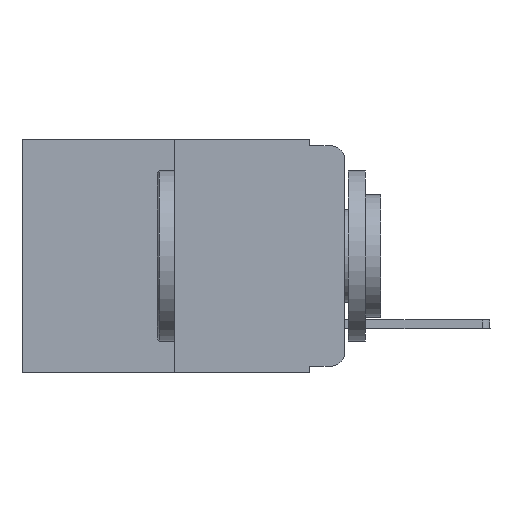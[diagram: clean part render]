
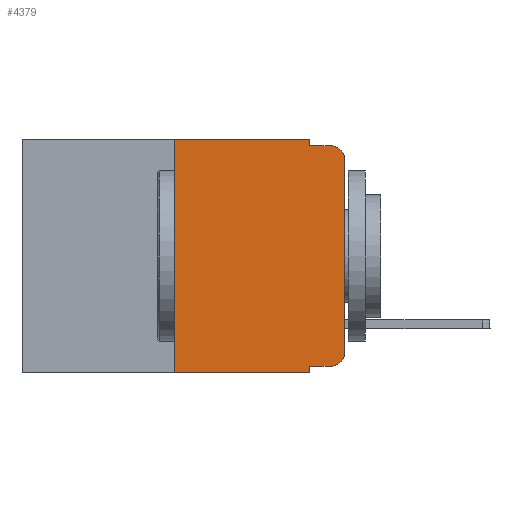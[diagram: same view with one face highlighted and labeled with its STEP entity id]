
A CAD part, left-side view. The second image highlights one B-rep face of the part: STEP entity #4379.
In plain terms, the highlighted planar face has unit normal (-1, 0, 0).
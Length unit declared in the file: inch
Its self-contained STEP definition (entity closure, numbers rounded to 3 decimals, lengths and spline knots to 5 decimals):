
#261 = DIRECTION ( 'NONE',  ( -1., 0., 0. ) ) ;
#300 = CARTESIAN_POINT ( 'NONE',  ( 0., 0.25, 0. ) ) ;
#353 = EDGE_CURVE ( 'NONE', #5328, #11144, #6289, .T. ) ;
#721 = VERTEX_POINT ( 'NONE', #13155 ) ;
#732 = LINE ( 'NONE', #4503, #10859 ) ;
#822 = ORIENTED_EDGE ( 'NONE', *, *, #2359, .T. ) ;
#826 = CARTESIAN_POINT ( 'NONE',  ( 0., 0.051, -0.01 ) ) ;
#854 = DIRECTION ( 'NONE',  ( 0., 0., -1. ) ) ;
#1128 = LINE ( 'NONE', #4908, #9444 ) ;
#1328 = DIRECTION ( 'NONE',  ( 0., 0., -1. ) ) ;
#1804 = VECTOR ( 'NONE', #5102, 39.37008 ) ;
#1822 = CARTESIAN_POINT ( 'NONE',  ( 0., 0.051, 0. ) ) ;
#1845 = FACE_OUTER_BOUND ( 'NONE', #6789, .T. ) ;
#1897 = DIRECTION ( 'NONE',  ( -1., 0., 0. ) ) ;
#2022 = VERTEX_POINT ( 'NONE', #10304 ) ;
#2359 = EDGE_CURVE ( 'NONE', #3665, #721, #9091, .T. ) ;
#2827 = ORIENTED_EDGE ( 'NONE', *, *, #7366, .F. ) ;
#2934 = DIRECTION ( 'NONE',  ( 0., 0., -1. ) ) ;
#3153 = VECTOR ( 'NONE', #10690, 39.37008 ) ;
#3536 = VECTOR ( 'NONE', #5840, 39.37008 ) ;
#3557 = CIRCLE ( 'NONE', #5397, 0.02 ) ;
#3665 = VERTEX_POINT ( 'NONE', #5564 ) ;
#3994 = DIRECTION ( 'NONE',  ( 1., 0., 0. ) ) ;
#4379 = ADVANCED_FACE ( 'NONE', ( #1845 ), #5975, .F. ) ;
#4503 = CARTESIAN_POINT ( 'NONE',  ( 0., 0.25, 0. ) ) ;
#4523 = DIRECTION ( 'NONE',  ( 0., -1., 0. ) ) ;
#4739 = CARTESIAN_POINT ( 'NONE',  ( 0., 0.051, 0. ) ) ;
#4783 = EDGE_CURVE ( 'NONE', #3665, #11144, #7653, .T. ) ;
#4908 = CARTESIAN_POINT ( 'NONE',  ( 0., 0., 0. ) ) ;
#5009 = CARTESIAN_POINT ( 'NONE',  ( 0., 0.051, -0.333 ) ) ;
#5102 = DIRECTION ( 'NONE',  ( 0., -1., 0. ) ) ;
#5114 = EDGE_CURVE ( 'NONE', #721, #13021, #11099, .T. ) ;
#5180 = CARTESIAN_POINT ( 'NONE',  ( 0., 0.473, 0. ) ) ;
#5328 = VERTEX_POINT ( 'NONE', #10017 ) ;
#5397 = AXIS2_PLACEMENT_3D ( 'NONE', #10200, #1897, #2934 ) ;
#5564 = CARTESIAN_POINT ( 'NONE',  ( 0., 0.051, -0.333 ) ) ;
#5840 = DIRECTION ( 'NONE',  ( 0., -1., 0. ) ) ;
#5975 = PLANE ( 'NONE',  #6290 ) ;
#6289 = LINE ( 'NONE', #8960, #3536 ) ;
#6290 = AXIS2_PLACEMENT_3D ( 'NONE', #5180, #3994, #854 ) ;
#6679 = EDGE_CURVE ( 'NONE', #7228, #2022, #3557, .T. ) ;
#6789 = EDGE_LOOP ( 'NONE', ( #12025, #11749, #9859, #8023, #7413, #2827, #7099, #11993, #822, #6969 ) ) ;
#6950 = CARTESIAN_POINT ( 'NONE',  ( 0., 0.051, -0.343 ) ) ;
#6969 = ORIENTED_EDGE ( 'NONE', *, *, #5114, .T. ) ;
#7013 = DIRECTION ( 'NONE',  ( 0., 0., 1. ) ) ;
#7099 = ORIENTED_EDGE ( 'NONE', *, *, #353, .T. ) ;
#7206 = VERTEX_POINT ( 'NONE', #1822 ) ;
#7228 = VERTEX_POINT ( 'NONE', #13267 ) ;
#7366 = EDGE_CURVE ( 'NONE', #5328, #9030, #732, .T. ) ;
#7413 = ORIENTED_EDGE ( 'NONE', *, *, #11383, .F. ) ;
#7653 = LINE ( 'NONE', #4739, #3153 ) ;
#7656 = EDGE_CURVE ( 'NONE', #9646, #2022, #9375, .T. ) ;
#8023 = ORIENTED_EDGE ( 'NONE', *, *, #13502, .F. ) ;
#8039 = CARTESIAN_POINT ( 'NONE',  ( 0., 0.02, -0.313 ) ) ;
#8700 = DIRECTION ( 'NONE',  ( 0., 0., 1. ) ) ;
#8789 = VECTOR ( 'NONE', #13421, 39.37008 ) ;
#8960 = CARTESIAN_POINT ( 'NONE',  ( 0., 0.473, -0.343 ) ) ;
#9030 = VERTEX_POINT ( 'NONE', #300 ) ;
#9080 = CARTESIAN_POINT ( 'NONE',  ( 0., 0.051, 0. ) ) ;
#9091 = LINE ( 'NONE', #5009, #1804 ) ;
#9375 = LINE ( 'NONE', #826, #10024 ) ;
#9444 = VECTOR ( 'NONE', #7013, 39.37008 ) ;
#9646 = VERTEX_POINT ( 'NONE', #11475 ) ;
#9859 = ORIENTED_EDGE ( 'NONE', *, *, #7656, .F. ) ;
#10017 = CARTESIAN_POINT ( 'NONE',  ( 0., 0.25, -0.343 ) ) ;
#10024 = VECTOR ( 'NONE', #13308, 39.37008 ) ;
#10200 = CARTESIAN_POINT ( 'NONE',  ( 0., 0.02, -0.03 ) ) ;
#10304 = CARTESIAN_POINT ( 'NONE',  ( 0., 0.02, -0.01 ) ) ;
#10405 = CARTESIAN_POINT ( 'NONE',  ( 0., 0., -0.313 ) ) ;
#10574 = EDGE_CURVE ( 'NONE', #13021, #7228, #1128, .T. ) ;
#10690 = DIRECTION ( 'NONE',  ( 0., 0., -1. ) ) ;
#10777 = LINE ( 'NONE', #9080, #8789 ) ;
#10859 = VECTOR ( 'NONE', #8700, 39.37008 ) ;
#11099 = CIRCLE ( 'NONE', #13483, 0.02 ) ;
#11144 = VERTEX_POINT ( 'NONE', #6950 ) ;
#11253 = VECTOR ( 'NONE', #4523, 39.37008 ) ;
#11383 = EDGE_CURVE ( 'NONE', #9030, #7206, #12268, .T. ) ;
#11475 = CARTESIAN_POINT ( 'NONE',  ( 0., 0.051, -0.01 ) ) ;
#11749 = ORIENTED_EDGE ( 'NONE', *, *, #6679, .T. ) ;
#11993 = ORIENTED_EDGE ( 'NONE', *, *, #4783, .F. ) ;
#12022 = CARTESIAN_POINT ( 'NONE',  ( 0., 0.473, 0. ) ) ;
#12025 = ORIENTED_EDGE ( 'NONE', *, *, #10574, .T. ) ;
#12268 = LINE ( 'NONE', #12022, #11253 ) ;
#13021 = VERTEX_POINT ( 'NONE', #10405 ) ;
#13155 = CARTESIAN_POINT ( 'NONE',  ( 0., 0.02, -0.333 ) ) ;
#13267 = CARTESIAN_POINT ( 'NONE',  ( 0., 0., -0.03 ) ) ;
#13308 = DIRECTION ( 'NONE',  ( 0., -1., 0. ) ) ;
#13421 = DIRECTION ( 'NONE',  ( 0., 0., -1. ) ) ;
#13483 = AXIS2_PLACEMENT_3D ( 'NONE', #8039, #261, #1328 ) ;
#13502 = EDGE_CURVE ( 'NONE', #7206, #9646, #10777, .T. ) ;
